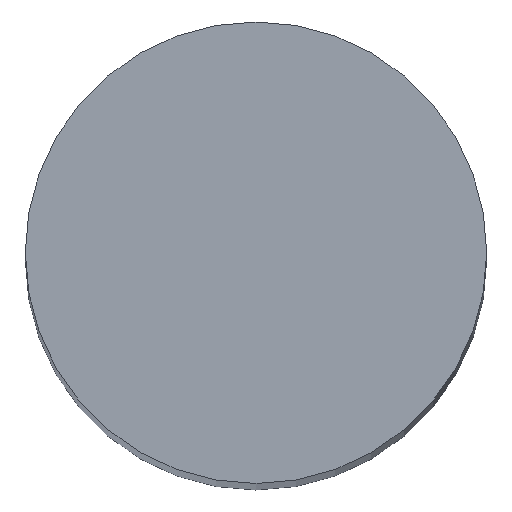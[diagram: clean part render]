
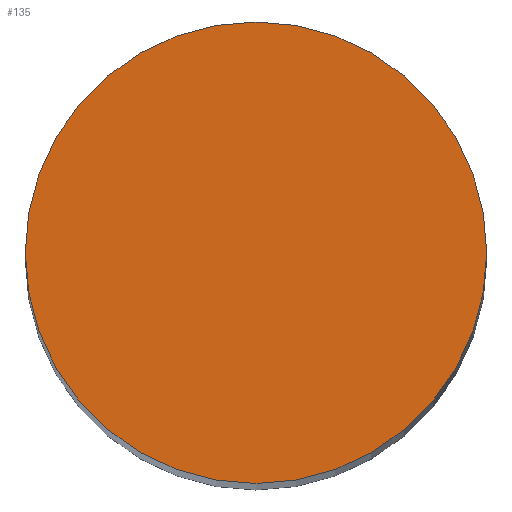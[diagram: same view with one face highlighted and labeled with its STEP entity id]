
A CAD part, top view. The second image highlights one B-rep face of the part: STEP entity #135.
In plain terms, the highlighted planar face has unit normal (0, 0, 1).
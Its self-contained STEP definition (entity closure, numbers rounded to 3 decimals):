
#6 = AXIS2_PLACEMENT_3D ( 'NONE', #19, #12, #27 ) ;
#12 = DIRECTION ( 'NONE',  ( 0., 0., 1. ) ) ;
#19 = CARTESIAN_POINT ( 'NONE',  ( 0., 0., 26.67 ) ) ;
#20 = CARTESIAN_POINT ( 'NONE',  ( 1.651, 0., 26.67 ) ) ;
#22 = DIRECTION ( 'NONE',  ( 1., 0., 0. ) ) ;
#26 = EDGE_CURVE ( 'NONE', #123, #137, #88, .T. ) ;
#27 = DIRECTION ( 'NONE',  ( 1., 0., 0. ) ) ;
#31 = EDGE_CURVE ( 'NONE', #137, #123, #91, .T. ) ;
#34 = DIRECTION ( 'NONE',  ( 0., 0., 1. ) ) ;
#44 = CARTESIAN_POINT ( 'NONE',  ( 0., 0., 26.67 ) ) ;
#46 = AXIS2_PLACEMENT_3D ( 'NONE', #44, #34, #22 ) ;
#53 = CARTESIAN_POINT ( 'NONE',  ( -1.651, 0., 26.67 ) ) ;
#57 = DIRECTION ( 'NONE',  ( 1., 0., 0. ) ) ;
#58 = DIRECTION ( 'NONE',  ( 0., 0., 1. ) ) ;
#62 = PLANE ( 'NONE',  #82 ) ;
#66 = FACE_OUTER_BOUND ( 'NONE', #111, .T. ) ;
#69 = CARTESIAN_POINT ( 'NONE',  ( 0., 0., 26.67 ) ) ;
#82 = AXIS2_PLACEMENT_3D ( 'NONE', #69, #58, #57 ) ;
#88 = CIRCLE ( 'NONE', #46, 1.651 ) ;
#91 = CIRCLE ( 'NONE', #6, 1.651 ) ;
#97 = ORIENTED_EDGE ( 'NONE', *, *, #31, .T. ) ;
#102 = ORIENTED_EDGE ( 'NONE', *, *, #26, .T. ) ;
#111 = EDGE_LOOP ( 'NONE', ( #97, #102 ) ) ;
#123 = VERTEX_POINT ( 'NONE', #20 ) ;
#135 = ADVANCED_FACE ( 'NONE', ( #66 ), #62, .T. ) ;
#137 = VERTEX_POINT ( 'NONE', #53 ) ;
